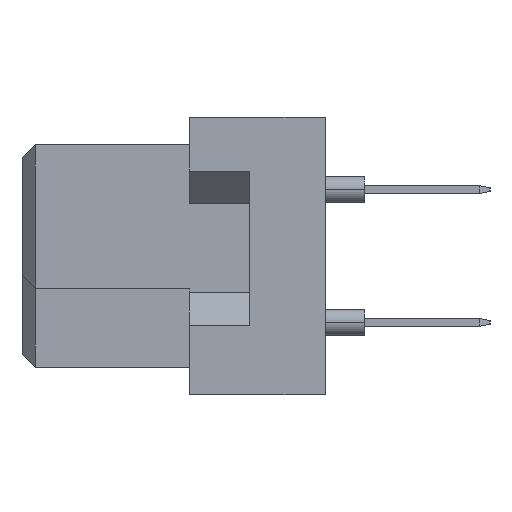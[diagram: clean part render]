
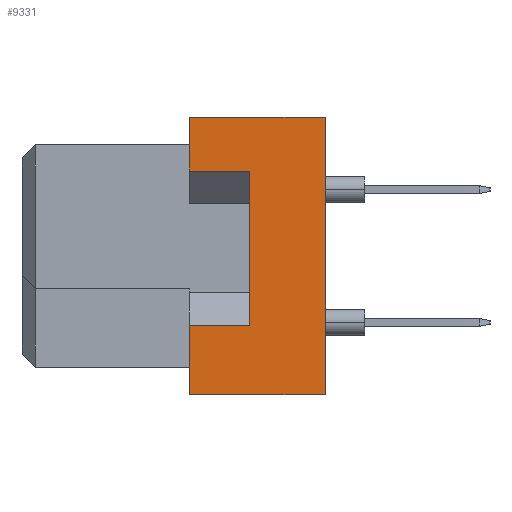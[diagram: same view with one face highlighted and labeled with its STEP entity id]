
A CAD part, left-side view. The second image highlights one B-rep face of the part: STEP entity #9331.
In plain terms, the highlighted planar face has unit normal (-1, 0, 0).
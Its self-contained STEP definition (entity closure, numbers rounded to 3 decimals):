
#570 = DIRECTION ( 'NONE',  ( 0., 1., 0. ) ) ;
#645 = VERTEX_POINT ( 'NONE', #2026 ) ;
#1136 = CARTESIAN_POINT ( 'NONE',  ( -27.5, -8.7, 3.25 ) ) ;
#1325 = CARTESIAN_POINT ( 'NONE',  ( -27.5, -6.4, -2.65 ) ) ;
#1335 = ORIENTED_EDGE ( 'NONE', *, *, #8278, .T. ) ;
#1797 = EDGE_CURVE ( 'NONE', #8897, #12160, #6793, .T. ) ;
#1829 = CARTESIAN_POINT ( 'NONE',  ( -27.5, -8.7, 3.25 ) ) ;
#2026 = CARTESIAN_POINT ( 'NONE',  ( -27.5, -6.4, 5.3 ) ) ;
#2069 = VECTOR ( 'NONE', #11647, 1000. ) ;
#2238 = ORIENTED_EDGE ( 'NONE', *, *, #1797, .F. ) ;
#2798 = LINE ( 'NONE', #7251, #6367 ) ;
#2932 = ORIENTED_EDGE ( 'NONE', *, *, #6547, .F. ) ;
#2998 = CARTESIAN_POINT ( 'NONE',  ( -27.5, -11.6, 5.3 ) ) ;
#3423 = EDGE_CURVE ( 'NONE', #7852, #14609, #8319, .T. ) ;
#4356 = DIRECTION ( 'NONE',  ( -1., 0., 0. ) ) ;
#4421 = ORIENTED_EDGE ( 'NONE', *, *, #6984, .F. ) ;
#4521 = VECTOR ( 'NONE', #570, 1000. ) ;
#4548 = VECTOR ( 'NONE', #5274, 1000. ) ;
#4757 = FACE_OUTER_BOUND ( 'NONE', #19667, .T. ) ;
#5274 = DIRECTION ( 'NONE',  ( 0., 1., 0. ) ) ;
#5332 = CARTESIAN_POINT ( 'NONE',  ( -27.5, -8.7, -2.65 ) ) ;
#5697 = DIRECTION ( 'NONE',  ( 0., 0., 1. ) ) ;
#6327 = VERTEX_POINT ( 'NONE', #19734 ) ;
#6367 = VECTOR ( 'NONE', #5697, 1000. ) ;
#6434 = CARTESIAN_POINT ( 'NONE',  ( -27.5, -11.6, -5.3 ) ) ;
#6508 = DIRECTION ( 'NONE',  ( 0., 0., 1. ) ) ;
#6547 = EDGE_CURVE ( 'NONE', #7852, #12063, #16826, .T. ) ;
#6793 = LINE ( 'NONE', #16233, #4521 ) ;
#6984 = EDGE_CURVE ( 'NONE', #12160, #14609, #9424, .T. ) ;
#7251 = CARTESIAN_POINT ( 'NONE',  ( -27.5, -6.4, -5.3 ) ) ;
#7294 = VECTOR ( 'NONE', #6508, 1000. ) ;
#7852 = VERTEX_POINT ( 'NONE', #19093 ) ;
#7955 = PLANE ( 'NONE',  #19878 ) ;
#8278 = EDGE_CURVE ( 'NONE', #6327, #645, #19480, .T. ) ;
#8319 = LINE ( 'NONE', #5332, #2069 ) ;
#8897 = VERTEX_POINT ( 'NONE', #6434 ) ;
#9331 = ADVANCED_FACE ( 'NONE', ( #4757 ), #7955, .T. ) ;
#9424 = LINE ( 'NONE', #9631, #7294 ) ;
#9631 = CARTESIAN_POINT ( 'NONE',  ( -27.5, -6.4, -5.3 ) ) ;
#9705 = DIRECTION ( 'NONE',  ( 0., 1., 0. ) ) ;
#9970 = ORIENTED_EDGE ( 'NONE', *, *, #3423, .T. ) ;
#10311 = VECTOR ( 'NONE', #20440, 1000. ) ;
#10574 = ORIENTED_EDGE ( 'NONE', *, *, #18353, .T. ) ;
#10782 = CARTESIAN_POINT ( 'NONE',  ( -27.5, -6.4, 3.25 ) ) ;
#11117 = EDGE_CURVE ( 'NONE', #12063, #13086, #11358, .T. ) ;
#11358 = LINE ( 'NONE', #1829, #11974 ) ;
#11405 = DIRECTION ( 'NONE',  ( 0., 0., 1. ) ) ;
#11490 = CARTESIAN_POINT ( 'NONE',  ( -27.5, -11.6, 5.3 ) ) ;
#11647 = DIRECTION ( 'NONE',  ( 0., 1., 0. ) ) ;
#11974 = VECTOR ( 'NONE', #9705, 1000. ) ;
#12063 = VERTEX_POINT ( 'NONE', #1136 ) ;
#12160 = VERTEX_POINT ( 'NONE', #14558 ) ;
#13086 = VERTEX_POINT ( 'NONE', #10782 ) ;
#13377 = ORIENTED_EDGE ( 'NONE', *, *, #20498, .F. ) ;
#14558 = CARTESIAN_POINT ( 'NONE',  ( -27.5, -6.4, -5.3 ) ) ;
#14609 = VERTEX_POINT ( 'NONE', #1325 ) ;
#15034 = VECTOR ( 'NONE', #11405, 1000. ) ;
#15767 = CARTESIAN_POINT ( 'NONE',  ( -27.5, -8.7, -2.65 ) ) ;
#16233 = CARTESIAN_POINT ( 'NONE',  ( -27.5, -11.6, -5.3 ) ) ;
#16260 = ORIENTED_EDGE ( 'NONE', *, *, #11117, .F. ) ;
#16826 = LINE ( 'NONE', #15767, #10311 ) ;
#18353 = EDGE_CURVE ( 'NONE', #8897, #6327, #19287, .T. ) ;
#18662 = DIRECTION ( 'NONE',  ( 0., 0., 1. ) ) ;
#19093 = CARTESIAN_POINT ( 'NONE',  ( -27.5, -8.7, -2.65 ) ) ;
#19178 = CARTESIAN_POINT ( 'NONE',  ( -27.5, -11.6, 5.3 ) ) ;
#19287 = LINE ( 'NONE', #19178, #15034 ) ;
#19480 = LINE ( 'NONE', #11490, #4548 ) ;
#19667 = EDGE_LOOP ( 'NONE', ( #9970, #4421, #2238, #10574, #1335, #13377, #16260, #2932 ) ) ;
#19734 = CARTESIAN_POINT ( 'NONE',  ( -27.5, -11.6, 5.3 ) ) ;
#19878 = AXIS2_PLACEMENT_3D ( 'NONE', #2998, #4356, #18662 ) ;
#20440 = DIRECTION ( 'NONE',  ( 0., 0., 1. ) ) ;
#20498 = EDGE_CURVE ( 'NONE', #13086, #645, #2798, .T. ) ;
